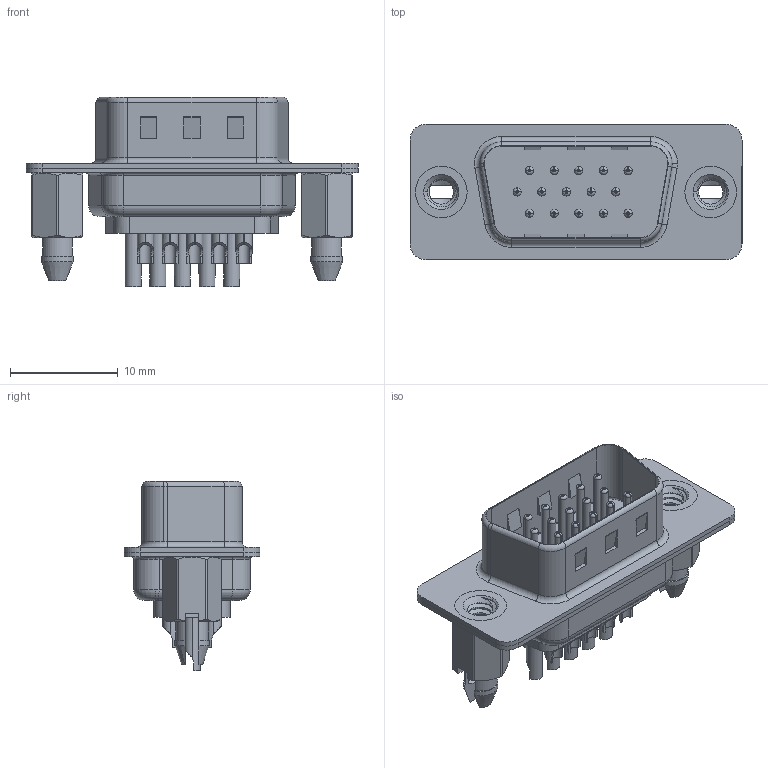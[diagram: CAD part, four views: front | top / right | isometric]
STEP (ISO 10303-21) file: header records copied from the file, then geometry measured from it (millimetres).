
FILE_DESCRIPTION (( 'STEP AP203' ), '1' );
FILE_NAME ('637-015-632-066.STEP', '2020-07-17T23:57:17', ( '' ), ( '' ), 'SwSTEP 2.0', 'SolidWorks 2020', '' );
FILE_SCHEMA (( 'CONFIG_CONTROL_DESIGN' ));
Length unit declared in the file: millimetre
Products named in the file (8): 637 Contact Row 2_32; 637 Contact Row 3_32; 637 Contact Row 1_32; 637 Shell Rear_15 Contacts; 637 Shell Front_15 Contacts; 637 Housing_15 Contacts; 637-015-632-066; 637 4-40 Threaded Boardlock_LP
Assembly tree (20 placements, depth 2):
  637-015-632-066
    637 Housing_15 Contacts
    637 Shell Front_15 Contacts
    637 Shell Rear_15 Contacts
    637 Contact Row 1_32  x5
    637 Contact Row 2_32  x5
    637 Contact Row 3_32  x5
    637 4-40 Threaded Boardlock_LP  x2
Bounding box: 30.8 x 12.6 x 17.55 mm (x, y, z)
Volume: 1444.2 mm3; surface area: 5064.2 mm2
Topology: 20 solids, 20 shells, 1338 faces, 3449 edges, 2190 vertices
Faces by surface type: cylinder 596, torus 365, plane 349, cone 22, bspline 6
Entity records: 20646 total; most frequent: CARTESIAN_POINT 4644, DIRECTION 3333, ORIENTED_EDGE 3000, EDGE_CURVE 1500, AXIS2_PLACEMENT_3D 1343, VERTEX_POINT 956, CIRCLE 727, EDGE_LOOP 690
